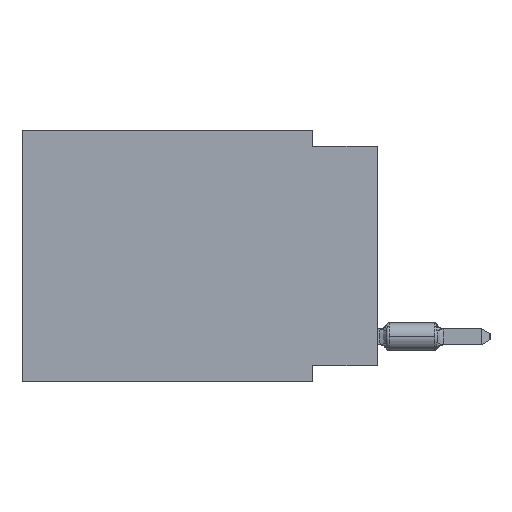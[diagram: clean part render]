
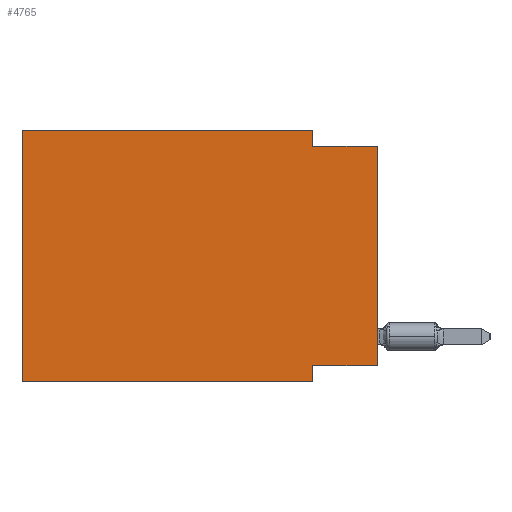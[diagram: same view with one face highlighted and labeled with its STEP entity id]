
A CAD part, left-side view. The second image highlights one B-rep face of the part: STEP entity #4765.
In plain terms, the highlighted planar face has unit normal (-1, 0, 0).
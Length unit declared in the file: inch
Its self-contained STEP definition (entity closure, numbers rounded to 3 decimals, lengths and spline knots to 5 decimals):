
#352 = LINE ( 'NONE', #2729, #8422 ) ;
#909 = LINE ( 'NONE', #31727, #3588 ) ;
#1244 = LINE ( 'NONE', #32259, #14997 ) ;
#1575 = ORIENTED_EDGE ( 'NONE', *, *, #3473, .F. ) ;
#2381 = EDGE_CURVE ( 'NONE', #35484, #5486, #909, .T. ) ;
#2614 = DIRECTION ( 'NONE',  ( 0., 0., -1. ) ) ;
#2645 = DIRECTION ( 'NONE',  ( 0., 1., 0. ) ) ;
#2729 = CARTESIAN_POINT ( 'NONE',  ( 0., 0., -0.025 ) ) ;
#2772 = LINE ( 'NONE', #27239, #10111 ) ;
#2929 = LINE ( 'NONE', #16801, #23966 ) ;
#3473 = EDGE_CURVE ( 'NONE', #18463, #20342, #30520, .T. ) ;
#3588 = VECTOR ( 'NONE', #31195, 39.37008 ) ;
#4765 = ADVANCED_FACE ( 'NONE', ( #13759 ), #22510, .F. ) ;
#4771 = VERTEX_POINT ( 'NONE', #30880 ) ;
#5161 = VERTEX_POINT ( 'NONE', #21018 ) ;
#5403 = VECTOR ( 'NONE', #2614, 39.37008 ) ;
#5486 = VERTEX_POINT ( 'NONE', #32473 ) ;
#5538 = CARTESIAN_POINT ( 'NONE',  ( 0., 0.55, 0. ) ) ;
#5629 = VECTOR ( 'NONE', #2645, 39.37008 ) ;
#6486 = CARTESIAN_POINT ( 'NONE',  ( 0., 0., -0.365 ) ) ;
#6792 = EDGE_LOOP ( 'NONE', ( #9975, #19117, #1575, #21919, #28038, #33547, #32044, #30705 ) ) ;
#8422 = VECTOR ( 'NONE', #22431, 39.37008 ) ;
#9975 = ORIENTED_EDGE ( 'NONE', *, *, #22850, .T. ) ;
#10111 = VECTOR ( 'NONE', #13907, 39.37008 ) ;
#10308 = CARTESIAN_POINT ( 'NONE',  ( 0., 0.1, 0. ) ) ;
#11658 = CARTESIAN_POINT ( 'NONE',  ( 0., 0.1, 0. ) ) ;
#11877 = CARTESIAN_POINT ( 'NONE',  ( 0., 0.55, -0.39 ) ) ;
#12221 = EDGE_CURVE ( 'NONE', #4771, #5486, #2772, .T. ) ;
#13759 = FACE_OUTER_BOUND ( 'NONE', #6792, .T. ) ;
#13907 = DIRECTION ( 'NONE',  ( 0., 0., -1. ) ) ;
#14508 = LINE ( 'NONE', #34016, #32088 ) ;
#14997 = VECTOR ( 'NONE', #20591, 39.37008 ) ;
#15040 = EDGE_CURVE ( 'NONE', #20342, #5161, #352, .T. ) ;
#16261 = DIRECTION ( 'NONE',  ( 0., -1., 0. ) ) ;
#16801 = CARTESIAN_POINT ( 'NONE',  ( 0., 0.55, 0. ) ) ;
#17447 = EDGE_CURVE ( 'NONE', #28249, #4771, #32753, .T. ) ;
#18463 = VERTEX_POINT ( 'NONE', #11658 ) ;
#18547 = EDGE_CURVE ( 'NONE', #35484, #24058, #1244, .T. ) ;
#18908 = AXIS2_PLACEMENT_3D ( 'NONE', #5538, #19236, #24878 ) ;
#19117 = ORIENTED_EDGE ( 'NONE', *, *, #15040, .F. ) ;
#19236 = DIRECTION ( 'NONE',  ( 1., 0., 0. ) ) ;
#20342 = VERTEX_POINT ( 'NONE', #33479 ) ;
#20591 = DIRECTION ( 'NONE',  ( 0., 0., 1. ) ) ;
#21018 = CARTESIAN_POINT ( 'NONE',  ( 0., 0., -0.025 ) ) ;
#21919 = ORIENTED_EDGE ( 'NONE', *, *, #23393, .F. ) ;
#22431 = DIRECTION ( 'NONE',  ( 0., -1., 0. ) ) ;
#22510 = PLANE ( 'NONE',  #18908 ) ;
#22850 = EDGE_CURVE ( 'NONE', #28249, #5161, #14508, .T. ) ;
#23393 = EDGE_CURVE ( 'NONE', #24058, #18463, #2929, .T. ) ;
#23966 = VECTOR ( 'NONE', #16261, 39.37008 ) ;
#24058 = VERTEX_POINT ( 'NONE', #28750 ) ;
#24878 = DIRECTION ( 'NONE',  ( 0., 0., -1. ) ) ;
#27239 = CARTESIAN_POINT ( 'NONE',  ( 0., 0.1, -0.39 ) ) ;
#27641 = CARTESIAN_POINT ( 'NONE',  ( 0., 0., -0.365 ) ) ;
#28038 = ORIENTED_EDGE ( 'NONE', *, *, #18547, .F. ) ;
#28249 = VERTEX_POINT ( 'NONE', #6486 ) ;
#28750 = CARTESIAN_POINT ( 'NONE',  ( 0., 0.55, 0. ) ) ;
#30520 = LINE ( 'NONE', #10308, #5403 ) ;
#30705 = ORIENTED_EDGE ( 'NONE', *, *, #17447, .F. ) ;
#30880 = CARTESIAN_POINT ( 'NONE',  ( 0., 0.1, -0.365 ) ) ;
#31195 = DIRECTION ( 'NONE',  ( 0., -1., 0. ) ) ;
#31280 = DIRECTION ( 'NONE',  ( 0., 0., 1. ) ) ;
#31727 = CARTESIAN_POINT ( 'NONE',  ( 0., 0.55, -0.39 ) ) ;
#32044 = ORIENTED_EDGE ( 'NONE', *, *, #12221, .F. ) ;
#32088 = VECTOR ( 'NONE', #31280, 39.37008 ) ;
#32259 = CARTESIAN_POINT ( 'NONE',  ( 0., 0.55, 0. ) ) ;
#32473 = CARTESIAN_POINT ( 'NONE',  ( 0., 0.1, -0.39 ) ) ;
#32753 = LINE ( 'NONE', #27641, #5629 ) ;
#33479 = CARTESIAN_POINT ( 'NONE',  ( 0., 0.1, -0.025 ) ) ;
#33547 = ORIENTED_EDGE ( 'NONE', *, *, #2381, .T. ) ;
#34016 = CARTESIAN_POINT ( 'NONE',  ( 0., 0., 0. ) ) ;
#35484 = VERTEX_POINT ( 'NONE', #11877 ) ;
